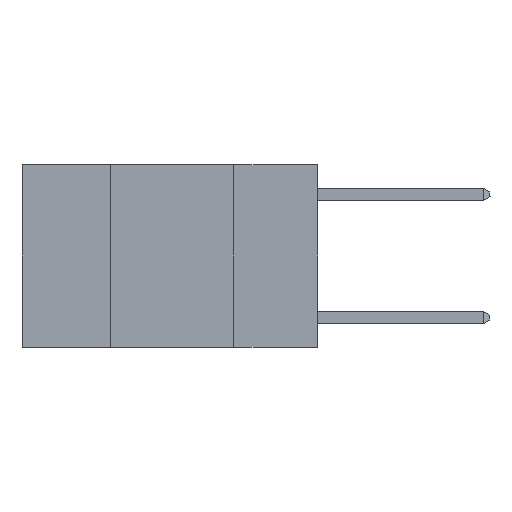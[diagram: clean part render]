
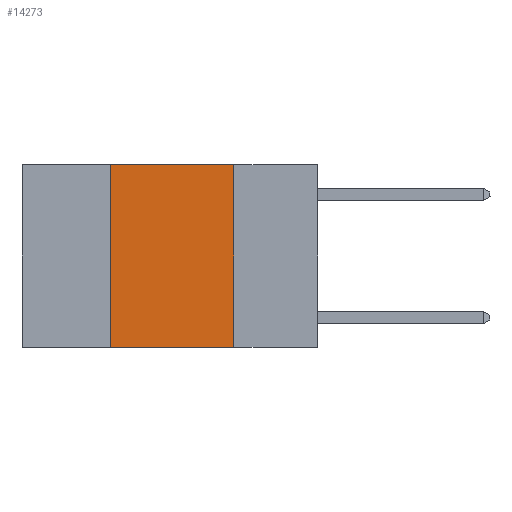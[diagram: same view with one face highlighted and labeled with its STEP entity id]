
A CAD part, left-side view. The second image highlights one B-rep face of the part: STEP entity #14273.
In plain terms, the highlighted planar face has unit normal (-1, 0, 0).
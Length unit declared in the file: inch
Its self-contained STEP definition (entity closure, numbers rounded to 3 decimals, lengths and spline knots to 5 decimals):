
#1216 = EDGE_CURVE ( 'NONE', #9868, #19413, #23943, .T. ) ;
#2620 = LINE ( 'NONE', #10813, #13192 ) ;
#2782 = PLANE ( 'NONE',  #19703 ) ;
#3224 = CARTESIAN_POINT ( 'NONE',  ( 0., 0.6, 0. ) ) ;
#3869 = CARTESIAN_POINT ( 'NONE',  ( 0., 0.42, -0.37 ) ) ;
#4192 = CARTESIAN_POINT ( 'NONE',  ( 0., 0.17, 0. ) ) ;
#4904 = DIRECTION ( 'NONE',  ( 0., 0., -1. ) ) ;
#5382 = EDGE_CURVE ( 'NONE', #20468, #19647, #10055, .T. ) ;
#6786 = VECTOR ( 'NONE', #22976, 39.37008 ) ;
#9700 = DIRECTION ( 'NONE',  ( 0., -1., 0. ) ) ;
#9868 = VERTEX_POINT ( 'NONE', #15290 ) ;
#10055 = LINE ( 'NONE', #21833, #14997 ) ;
#10813 = CARTESIAN_POINT ( 'NONE',  ( 0., 0.42, 0. ) ) ;
#11427 = DIRECTION ( 'NONE',  ( 0., -1., 0. ) ) ;
#13192 = VECTOR ( 'NONE', #17113, 39.37008 ) ;
#13312 = CARTESIAN_POINT ( 'NONE',  ( 0., 0.6, 0. ) ) ;
#13330 = EDGE_CURVE ( 'NONE', #19413, #19647, #17928, .T. ) ;
#14273 = ADVANCED_FACE ( 'NONE', ( #17236 ), #2782, .F. ) ;
#14997 = VECTOR ( 'NONE', #11427, 39.37008 ) ;
#15290 = CARTESIAN_POINT ( 'NONE',  ( 0., 0.42, 0. ) ) ;
#17113 = DIRECTION ( 'NONE',  ( 0., 0., 1. ) ) ;
#17236 = FACE_OUTER_BOUND ( 'NONE', #18164, .T. ) ;
#17496 = DIRECTION ( 'NONE',  ( 1., 0., 0. ) ) ;
#17928 = LINE ( 'NONE', #4192, #6786 ) ;
#18164 = EDGE_LOOP ( 'NONE', ( #24825, #20620, #23875, #27032 ) ) ;
#18396 = VECTOR ( 'NONE', #9700, 39.37008 ) ;
#19413 = VERTEX_POINT ( 'NONE', #23630 ) ;
#19647 = VERTEX_POINT ( 'NONE', #24480 ) ;
#19703 = AXIS2_PLACEMENT_3D ( 'NONE', #13312, #17496, #4904 ) ;
#20468 = VERTEX_POINT ( 'NONE', #3869 ) ;
#20620 = ORIENTED_EDGE ( 'NONE', *, *, #1216, .F. ) ;
#21833 = CARTESIAN_POINT ( 'NONE',  ( 0., 0.6, -0.37 ) ) ;
#22976 = DIRECTION ( 'NONE',  ( 0., 0., -1. ) ) ;
#23630 = CARTESIAN_POINT ( 'NONE',  ( 0., 0.17, 0. ) ) ;
#23810 = EDGE_CURVE ( 'NONE', #20468, #9868, #2620, .T. ) ;
#23875 = ORIENTED_EDGE ( 'NONE', *, *, #23810, .F. ) ;
#23943 = LINE ( 'NONE', #3224, #18396 ) ;
#24480 = CARTESIAN_POINT ( 'NONE',  ( 0., 0.17, -0.37 ) ) ;
#24825 = ORIENTED_EDGE ( 'NONE', *, *, #13330, .F. ) ;
#27032 = ORIENTED_EDGE ( 'NONE', *, *, #5382, .T. ) ;
